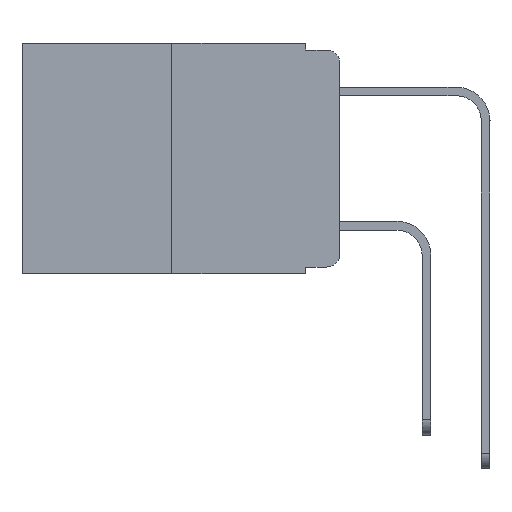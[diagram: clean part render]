
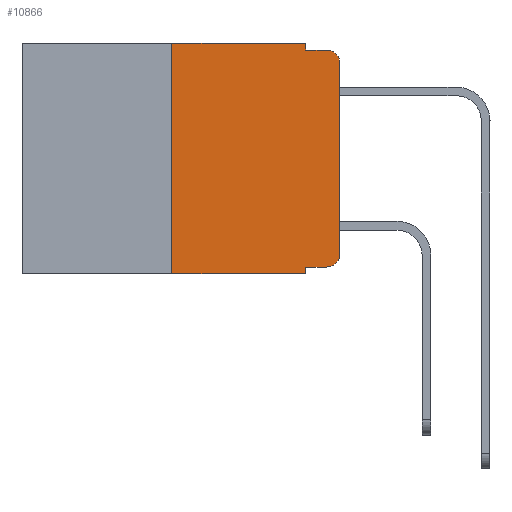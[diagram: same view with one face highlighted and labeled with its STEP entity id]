
A CAD part, left-side view. The second image highlights one B-rep face of the part: STEP entity #10866.
In plain terms, the highlighted planar face has unit normal (-1, 0, 0).
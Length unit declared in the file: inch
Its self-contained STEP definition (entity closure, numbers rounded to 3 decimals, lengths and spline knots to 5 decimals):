
#78 = EDGE_LOOP ( 'NONE', ( #23321, #21871, #18019, #8445, #14139, #4423, #24783, #5047, #958, #7524 ) ) ;
#603 = DIRECTION ( 'NONE',  ( 0., -1., 0. ) ) ;
#857 = VERTEX_POINT ( 'NONE', #9049 ) ;
#941 = EDGE_CURVE ( 'NONE', #22352, #24306, #17473, .T. ) ;
#958 = ORIENTED_EDGE ( 'NONE', *, *, #12932, .T. ) ;
#1145 = VERTEX_POINT ( 'NONE', #5109 ) ;
#1539 = VERTEX_POINT ( 'NONE', #7170 ) ;
#1753 = VECTOR ( 'NONE', #8386, 39.37008 ) ;
#1956 = VECTOR ( 'NONE', #19183, 39.37008 ) ;
#2319 = CARTESIAN_POINT ( 'NONE',  ( 0., 0.25, 0. ) ) ;
#2395 = LINE ( 'NONE', #16023, #1753 ) ;
#2932 = VECTOR ( 'NONE', #603, 39.37008 ) ;
#3087 = VERTEX_POINT ( 'NONE', #18598 ) ;
#4295 = CARTESIAN_POINT ( 'NONE',  ( 0., 0.473, -0.343 ) ) ;
#4423 = ORIENTED_EDGE ( 'NONE', *, *, #14451, .F. ) ;
#4585 = VERTEX_POINT ( 'NONE', #7798 ) ;
#4612 = CIRCLE ( 'NONE', #12345, 0.02 ) ;
#4940 = VERTEX_POINT ( 'NONE', #5088 ) ;
#5047 = ORIENTED_EDGE ( 'NONE', *, *, #18331, .F. ) ;
#5088 = CARTESIAN_POINT ( 'NONE',  ( 0., 0.051, -0.333 ) ) ;
#5109 = CARTESIAN_POINT ( 'NONE',  ( 0., 0.02, -0.333 ) ) ;
#6450 = CIRCLE ( 'NONE', #18513, 0.02 ) ;
#7170 = CARTESIAN_POINT ( 'NONE',  ( 0., 0.051, -0.343 ) ) ;
#7208 = PLANE ( 'NONE',  #22468 ) ;
#7356 = CARTESIAN_POINT ( 'NONE',  ( 0., 0.02, -0.313 ) ) ;
#7440 = EDGE_CURVE ( 'NONE', #3087, #24306, #4612, .T. ) ;
#7524 = ORIENTED_EDGE ( 'NONE', *, *, #22034, .T. ) ;
#7645 = LINE ( 'NONE', #20194, #22311 ) ;
#7798 = CARTESIAN_POINT ( 'NONE',  ( 0., 0.051, 0. ) ) ;
#7954 = CARTESIAN_POINT ( 'NONE',  ( 0., 0.25, -0.343 ) ) ;
#8386 = DIRECTION ( 'NONE',  ( 0., 0., -1. ) ) ;
#8445 = ORIENTED_EDGE ( 'NONE', *, *, #9140, .F. ) ;
#8634 = DIRECTION ( 'NONE',  ( -1., 0., 0. ) ) ;
#8853 = CARTESIAN_POINT ( 'NONE',  ( 0., 0.051, -0.01 ) ) ;
#9049 = CARTESIAN_POINT ( 'NONE',  ( 0., 0., -0.313 ) ) ;
#9140 = EDGE_CURVE ( 'NONE', #4585, #22352, #20279, .T. ) ;
#9149 = DIRECTION ( 'NONE',  ( 0., 0., 1. ) ) ;
#9194 = DIRECTION ( 'NONE',  ( 1., 0., 0. ) ) ;
#9337 = DIRECTION ( 'NONE',  ( 0., 0., -1. ) ) ;
#10122 = EDGE_CURVE ( 'NONE', #23603, #4585, #17785, .T. ) ;
#10331 = CARTESIAN_POINT ( 'NONE',  ( 0., 0.051, -0.01 ) ) ;
#10866 = ADVANCED_FACE ( 'NONE', ( #16284 ), #7208, .F. ) ;
#11360 = DIRECTION ( 'NONE',  ( 0., 0., -1. ) ) ;
#11367 = DIRECTION ( 'NONE',  ( 0., 0., 1. ) ) ;
#12124 = DIRECTION ( 'NONE',  ( 0., -1., 0. ) ) ;
#12345 = AXIS2_PLACEMENT_3D ( 'NONE', #20124, #8634, #21979 ) ;
#12386 = CARTESIAN_POINT ( 'NONE',  ( 0., 0.473, 0. ) ) ;
#12581 = CARTESIAN_POINT ( 'NONE',  ( 0., 0.02, -0.01 ) ) ;
#12932 = EDGE_CURVE ( 'NONE', #4940, #1145, #7645, .T. ) ;
#13366 = VECTOR ( 'NONE', #11367, 39.37008 ) ;
#14139 = ORIENTED_EDGE ( 'NONE', *, *, #10122, .F. ) ;
#14451 = EDGE_CURVE ( 'NONE', #24156, #23603, #16014, .T. ) ;
#14482 = DIRECTION ( 'NONE',  ( 0., -1., 0. ) ) ;
#15303 = VECTOR ( 'NONE', #12124, 39.37008 ) ;
#16014 = LINE ( 'NONE', #20621, #20500 ) ;
#16023 = CARTESIAN_POINT ( 'NONE',  ( 0., 0.051, 0. ) ) ;
#16122 = EDGE_CURVE ( 'NONE', #24156, #1539, #20404, .T. ) ;
#16284 = FACE_OUTER_BOUND ( 'NONE', #78, .T. ) ;
#17473 = LINE ( 'NONE', #8853, #1956 ) ;
#17785 = LINE ( 'NONE', #12386, #2932 ) ;
#18019 = ORIENTED_EDGE ( 'NONE', *, *, #941, .F. ) ;
#18331 = EDGE_CURVE ( 'NONE', #4940, #1539, #2395, .T. ) ;
#18513 = AXIS2_PLACEMENT_3D ( 'NONE', #7356, #20809, #9337 ) ;
#18598 = CARTESIAN_POINT ( 'NONE',  ( 0., 0., -0.03 ) ) ;
#19052 = CARTESIAN_POINT ( 'NONE',  ( 0., 0., 0. ) ) ;
#19183 = DIRECTION ( 'NONE',  ( 0., -1., 0. ) ) ;
#19644 = LINE ( 'NONE', #19052, #13366 ) ;
#20124 = CARTESIAN_POINT ( 'NONE',  ( 0., 0.02, -0.03 ) ) ;
#20194 = CARTESIAN_POINT ( 'NONE',  ( 0., 0.051, -0.333 ) ) ;
#20279 = LINE ( 'NONE', #24614, #20864 ) ;
#20404 = LINE ( 'NONE', #4295, #15303 ) ;
#20500 = VECTOR ( 'NONE', #9149, 39.37008 ) ;
#20621 = CARTESIAN_POINT ( 'NONE',  ( 0., 0.25, 0. ) ) ;
#20672 = CARTESIAN_POINT ( 'NONE',  ( 0., 0.473, 0. ) ) ;
#20809 = DIRECTION ( 'NONE',  ( -1., 0., 0. ) ) ;
#20864 = VECTOR ( 'NONE', #11360, 39.37008 ) ;
#21871 = ORIENTED_EDGE ( 'NONE', *, *, #7440, .T. ) ;
#21979 = DIRECTION ( 'NONE',  ( 0., 0., -1. ) ) ;
#22034 = EDGE_CURVE ( 'NONE', #1145, #857, #6450, .T. ) ;
#22311 = VECTOR ( 'NONE', #14482, 39.37008 ) ;
#22352 = VERTEX_POINT ( 'NONE', #10331 ) ;
#22468 = AXIS2_PLACEMENT_3D ( 'NONE', #20672, #9194, #22531 ) ;
#22531 = DIRECTION ( 'NONE',  ( 0., 0., -1. ) ) ;
#23321 = ORIENTED_EDGE ( 'NONE', *, *, #23342, .T. ) ;
#23342 = EDGE_CURVE ( 'NONE', #857, #3087, #19644, .T. ) ;
#23603 = VERTEX_POINT ( 'NONE', #2319 ) ;
#24156 = VERTEX_POINT ( 'NONE', #7954 ) ;
#24306 = VERTEX_POINT ( 'NONE', #12581 ) ;
#24614 = CARTESIAN_POINT ( 'NONE',  ( 0., 0.051, 0. ) ) ;
#24783 = ORIENTED_EDGE ( 'NONE', *, *, #16122, .T. ) ;
